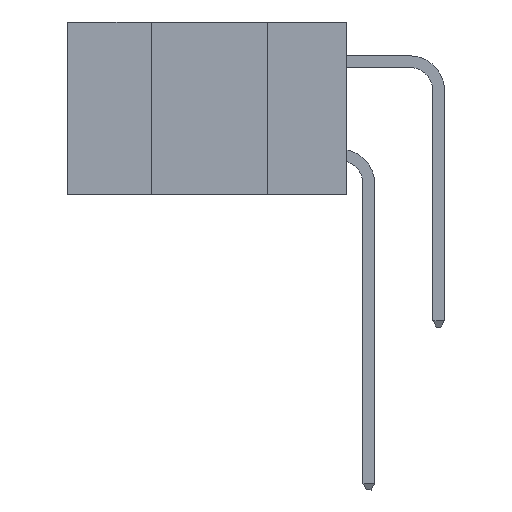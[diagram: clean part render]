
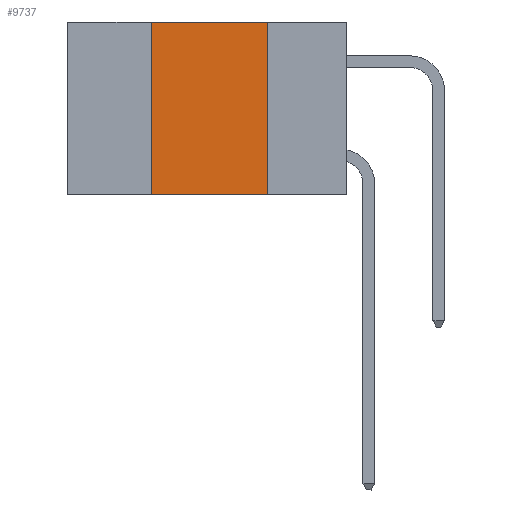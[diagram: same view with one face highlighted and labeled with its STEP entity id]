
A CAD part, left-side view. The second image highlights one B-rep face of the part: STEP entity #9737.
In plain terms, the highlighted planar face has unit normal (-1, 0, 0).
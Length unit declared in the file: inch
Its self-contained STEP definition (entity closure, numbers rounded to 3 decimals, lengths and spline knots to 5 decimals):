
#151 = ORIENTED_EDGE ( 'NONE', *, *, #1716, .F. ) ;
#353 = VECTOR ( 'NONE', #21256, 39.37008 ) ;
#1000 = CARTESIAN_POINT ( 'NONE',  ( 0., 0.6, 0. ) ) ;
#1001 = CARTESIAN_POINT ( 'NONE',  ( 0., 0.6, 0. ) ) ;
#1226 = VERTEX_POINT ( 'NONE', #13737 ) ;
#1257 = DIRECTION ( 'NONE',  ( 0., 0., 1. ) ) ;
#1716 = EDGE_CURVE ( 'NONE', #5622, #6013, #10681, .T. ) ;
#2348 = DIRECTION ( 'NONE',  ( 0., 0., -1. ) ) ;
#2828 = DIRECTION ( 'NONE',  ( 0., -1., 0. ) ) ;
#4817 = EDGE_LOOP ( 'NONE', ( #151, #6262, #11811, #8057 ) ) ;
#5622 = VERTEX_POINT ( 'NONE', #18489 ) ;
#6013 = VERTEX_POINT ( 'NONE', #11165 ) ;
#6105 = LINE ( 'NONE', #19788, #8473 ) ;
#6262 = ORIENTED_EDGE ( 'NONE', *, *, #7713, .F. ) ;
#6263 = VECTOR ( 'NONE', #2348, 39.37008 ) ;
#7713 = EDGE_CURVE ( 'NONE', #1226, #5622, #18322, .T. ) ;
#8057 = ORIENTED_EDGE ( 'NONE', *, *, #10869, .T. ) ;
#8473 = VECTOR ( 'NONE', #1257, 39.37008 ) ;
#9737 = ADVANCED_FACE ( 'NONE', ( #16417 ), #11583, .F. ) ;
#10681 = LINE ( 'NONE', #10899, #6263 ) ;
#10869 = EDGE_CURVE ( 'NONE', #17816, #6013, #11173, .T. ) ;
#10899 = CARTESIAN_POINT ( 'NONE',  ( 0., 0.17, 0. ) ) ;
#11165 = CARTESIAN_POINT ( 'NONE',  ( 0., 0.17, -0.37 ) ) ;
#11173 = LINE ( 'NONE', #14643, #353 ) ;
#11546 = CARTESIAN_POINT ( 'NONE',  ( 0., 0.42, -0.37 ) ) ;
#11583 = PLANE ( 'NONE',  #16117 ) ;
#11811 = ORIENTED_EDGE ( 'NONE', *, *, #20057, .F. ) ;
#13737 = CARTESIAN_POINT ( 'NONE',  ( 0., 0.42, 0. ) ) ;
#14643 = CARTESIAN_POINT ( 'NONE',  ( 0., 0.6, -0.37 ) ) ;
#14724 = DIRECTION ( 'NONE',  ( 0., 0., -1. ) ) ;
#15530 = VECTOR ( 'NONE', #2828, 39.37008 ) ;
#16117 = AXIS2_PLACEMENT_3D ( 'NONE', #1001, #18213, #14724 ) ;
#16417 = FACE_OUTER_BOUND ( 'NONE', #4817, .T. ) ;
#17816 = VERTEX_POINT ( 'NONE', #11546 ) ;
#18213 = DIRECTION ( 'NONE',  ( 1., 0., 0. ) ) ;
#18322 = LINE ( 'NONE', #1000, #15530 ) ;
#18489 = CARTESIAN_POINT ( 'NONE',  ( 0., 0.17, 0. ) ) ;
#19788 = CARTESIAN_POINT ( 'NONE',  ( 0., 0.42, 0. ) ) ;
#20057 = EDGE_CURVE ( 'NONE', #17816, #1226, #6105, .T. ) ;
#21256 = DIRECTION ( 'NONE',  ( 0., -1., 0. ) ) ;
